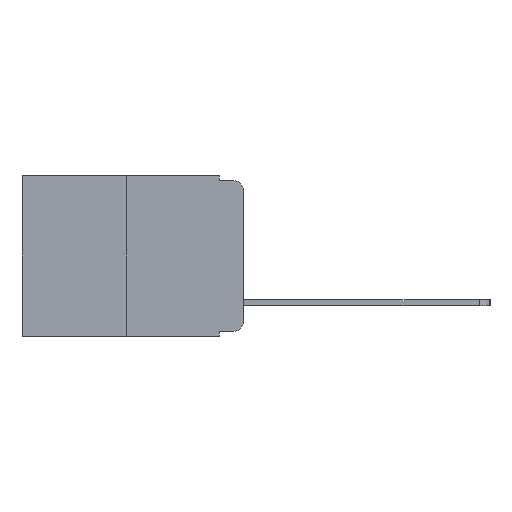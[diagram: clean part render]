
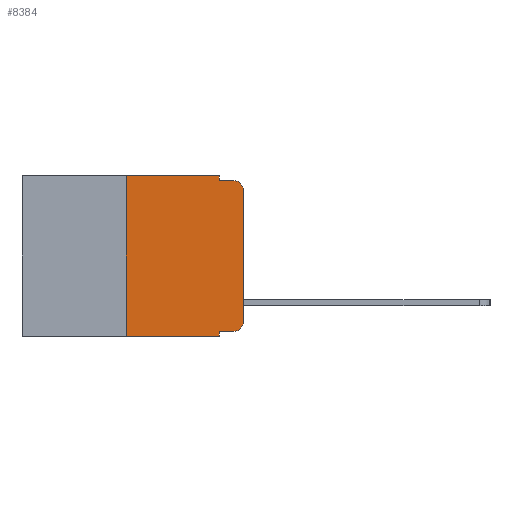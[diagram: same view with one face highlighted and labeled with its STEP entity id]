
A CAD part, left-side view. The second image highlights one B-rep face of the part: STEP entity #8384.
In plain terms, the highlighted planar face has unit normal (-1, 0, 0).
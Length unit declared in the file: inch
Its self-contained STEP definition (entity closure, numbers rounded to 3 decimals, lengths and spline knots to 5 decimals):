
#75 = VERTEX_POINT ( 'NONE', #7574 ) ;
#367 = CARTESIAN_POINT ( 'NONE',  ( 0., 0.051, 0. ) ) ;
#513 = ORIENTED_EDGE ( 'NONE', *, *, #13842, .F. ) ;
#940 = CARTESIAN_POINT ( 'NONE',  ( 0., 0., -0.313 ) ) ;
#1044 = EDGE_CURVE ( 'NONE', #10162, #8000, #9208, .T. ) ;
#1302 = LINE ( 'NONE', #2463, #7115 ) ;
#1552 = DIRECTION ( 'NONE',  ( 0., 0., -1. ) ) ;
#1698 = CARTESIAN_POINT ( 'NONE',  ( 0., 0.051, -0.01 ) ) ;
#1801 = CARTESIAN_POINT ( 'NONE',  ( 0., 0.051, -0.333 ) ) ;
#1866 = ORIENTED_EDGE ( 'NONE', *, *, #5791, .F. ) ;
#2043 = VERTEX_POINT ( 'NONE', #5090 ) ;
#2216 = DIRECTION ( 'NONE',  ( -1., 0., 0. ) ) ;
#2239 = VERTEX_POINT ( 'NONE', #1698 ) ;
#2463 = CARTESIAN_POINT ( 'NONE',  ( 0., 0.051, 0. ) ) ;
#2557 = VECTOR ( 'NONE', #13034, 39.37008 ) ;
#3093 = LINE ( 'NONE', #5191, #11909 ) ;
#3305 = LINE ( 'NONE', #10292, #9099 ) ;
#3539 = ORIENTED_EDGE ( 'NONE', *, *, #13226, .F. ) ;
#3663 = VERTEX_POINT ( 'NONE', #3732 ) ;
#3732 = CARTESIAN_POINT ( 'NONE',  ( 0., 0.02, -0.333 ) ) ;
#3832 = ORIENTED_EDGE ( 'NONE', *, *, #7000, .T. ) ;
#3948 = VERTEX_POINT ( 'NONE', #11084 ) ;
#4040 = DIRECTION ( 'NONE',  ( 0., 0., 1. ) ) ;
#4136 = AXIS2_PLACEMENT_3D ( 'NONE', #13022, #6157, #14154 ) ;
#4363 = VECTOR ( 'NONE', #6834, 39.37008 ) ;
#4525 = DIRECTION ( 'NONE',  ( 0., -1., 0. ) ) ;
#4665 = DIRECTION ( 'NONE',  ( 0., 0., -1. ) ) ;
#4780 = VECTOR ( 'NONE', #1552, 39.37008 ) ;
#5090 = CARTESIAN_POINT ( 'NONE',  ( 0., 0.051, 0. ) ) ;
#5191 = CARTESIAN_POINT ( 'NONE',  ( 0., 0.25, 0. ) ) ;
#5686 = EDGE_CURVE ( 'NONE', #3663, #10162, #11391, .T. ) ;
#5791 = EDGE_CURVE ( 'NONE', #8768, #3948, #3093, .T. ) ;
#6110 = ORIENTED_EDGE ( 'NONE', *, *, #12246, .F. ) ;
#6125 = VECTOR ( 'NONE', #12574, 39.37008 ) ;
#6157 = DIRECTION ( 'NONE',  ( -1., 0., 0. ) ) ;
#6834 = DIRECTION ( 'NONE',  ( 0., -1., 0. ) ) ;
#7000 = EDGE_CURVE ( 'NONE', #8768, #9346, #12101, .T. ) ;
#7115 = VECTOR ( 'NONE', #12808, 39.37008 ) ;
#7326 = ORIENTED_EDGE ( 'NONE', *, *, #11096, .T. ) ;
#7400 = VERTEX_POINT ( 'NONE', #10659 ) ;
#7429 = LINE ( 'NONE', #13672, #4363 ) ;
#7568 = CARTESIAN_POINT ( 'NONE',  ( 0., 0.051, -0.343 ) ) ;
#7574 = CARTESIAN_POINT ( 'NONE',  ( 0., 0.051, -0.333 ) ) ;
#7839 = EDGE_CURVE ( 'NONE', #8000, #7400, #9767, .T. ) ;
#8000 = VERTEX_POINT ( 'NONE', #12855 ) ;
#8106 = PLANE ( 'NONE',  #12331 ) ;
#8220 = LINE ( 'NONE', #367, #4780 ) ;
#8316 = AXIS2_PLACEMENT_3D ( 'NONE', #9141, #2216, #10302 ) ;
#8384 = ADVANCED_FACE ( 'NONE', ( #11000 ), #8106, .F. ) ;
#8509 = CARTESIAN_POINT ( 'NONE',  ( 0., 0.473, -0.343 ) ) ;
#8732 = ORIENTED_EDGE ( 'NONE', *, *, #12708, .F. ) ;
#8737 = DIRECTION ( 'NONE',  ( 0., -1., 0. ) ) ;
#8756 = CARTESIAN_POINT ( 'NONE',  ( 0., 0., 0. ) ) ;
#8768 = VERTEX_POINT ( 'NONE', #9966 ) ;
#8781 = ORIENTED_EDGE ( 'NONE', *, *, #5686, .T. ) ;
#8808 = VECTOR ( 'NONE', #8737, 39.37008 ) ;
#9099 = VECTOR ( 'NONE', #4525, 39.37008 ) ;
#9141 = CARTESIAN_POINT ( 'NONE',  ( 0., 0.02, -0.03 ) ) ;
#9208 = LINE ( 'NONE', #8756, #6125 ) ;
#9223 = CARTESIAN_POINT ( 'NONE',  ( 0., 0.473, 0. ) ) ;
#9346 = VERTEX_POINT ( 'NONE', #7568 ) ;
#9767 = CIRCLE ( 'NONE', #8316, 0.02 ) ;
#9954 = EDGE_LOOP ( 'NONE', ( #11145, #14014, #513, #8732, #3539, #1866, #3832, #6110, #7326, #8781 ) ) ;
#9966 = CARTESIAN_POINT ( 'NONE',  ( 0., 0.25, -0.343 ) ) ;
#10162 = VERTEX_POINT ( 'NONE', #940 ) ;
#10292 = CARTESIAN_POINT ( 'NONE',  ( 0., 0.473, 0. ) ) ;
#10302 = DIRECTION ( 'NONE',  ( 0., 0., -1. ) ) ;
#10659 = CARTESIAN_POINT ( 'NONE',  ( 0., 0.02, -0.01 ) ) ;
#11000 = FACE_OUTER_BOUND ( 'NONE', #9954, .T. ) ;
#11084 = CARTESIAN_POINT ( 'NONE',  ( 0., 0.25, 0. ) ) ;
#11096 = EDGE_CURVE ( 'NONE', #75, #3663, #14495, .T. ) ;
#11145 = ORIENTED_EDGE ( 'NONE', *, *, #1044, .T. ) ;
#11391 = CIRCLE ( 'NONE', #4136, 0.02 ) ;
#11552 = DIRECTION ( 'NONE',  ( 1., 0., 0. ) ) ;
#11909 = VECTOR ( 'NONE', #4040, 39.37008 ) ;
#12101 = LINE ( 'NONE', #8509, #2557 ) ;
#12246 = EDGE_CURVE ( 'NONE', #75, #9346, #8220, .T. ) ;
#12331 = AXIS2_PLACEMENT_3D ( 'NONE', #9223, #11552, #4665 ) ;
#12574 = DIRECTION ( 'NONE',  ( 0., 0., 1. ) ) ;
#12708 = EDGE_CURVE ( 'NONE', #2043, #2239, #1302, .T. ) ;
#12808 = DIRECTION ( 'NONE',  ( 0., 0., -1. ) ) ;
#12855 = CARTESIAN_POINT ( 'NONE',  ( 0., 0., -0.03 ) ) ;
#13022 = CARTESIAN_POINT ( 'NONE',  ( 0., 0.02, -0.313 ) ) ;
#13034 = DIRECTION ( 'NONE',  ( 0., -1., 0. ) ) ;
#13226 = EDGE_CURVE ( 'NONE', #3948, #2043, #3305, .T. ) ;
#13672 = CARTESIAN_POINT ( 'NONE',  ( 0., 0.051, -0.01 ) ) ;
#13842 = EDGE_CURVE ( 'NONE', #2239, #7400, #7429, .T. ) ;
#14014 = ORIENTED_EDGE ( 'NONE', *, *, #7839, .T. ) ;
#14154 = DIRECTION ( 'NONE',  ( 0., 0., -1. ) ) ;
#14495 = LINE ( 'NONE', #1801, #8808 ) ;
